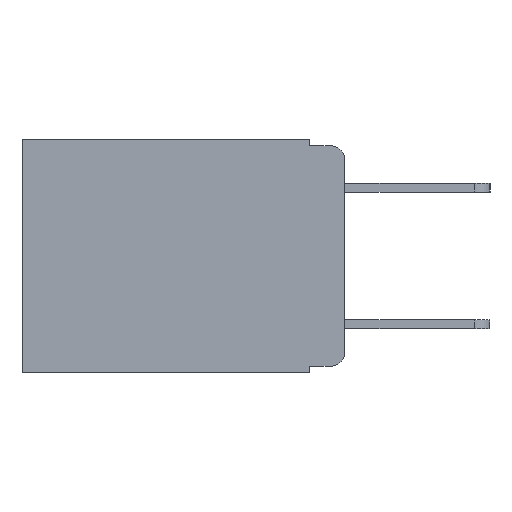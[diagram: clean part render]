
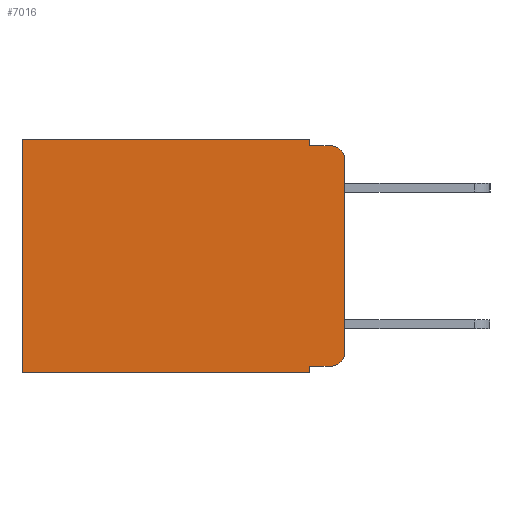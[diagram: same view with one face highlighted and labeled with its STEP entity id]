
A CAD part, left-side view. The second image highlights one B-rep face of the part: STEP entity #7016.
In plain terms, the highlighted planar face has unit normal (-1, 0, 0).
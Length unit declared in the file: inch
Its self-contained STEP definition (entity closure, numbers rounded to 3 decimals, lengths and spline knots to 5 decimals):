
#31 = ORIENTED_EDGE ( 'NONE', *, *, #5217, .T. ) ;
#82 = CARTESIAN_POINT ( 'NONE',  ( 0.298, 0.051, -0.343 ) ) ;
#158 = ORIENTED_EDGE ( 'NONE', *, *, #9472, .F. ) ;
#251 = ORIENTED_EDGE ( 'NONE', *, *, #9410, .F. ) ;
#436 = VERTEX_POINT ( 'NONE', #82 ) ;
#536 = ORIENTED_EDGE ( 'NONE', *, *, #9461, .T. ) ;
#599 = ORIENTED_EDGE ( 'NONE', *, *, #13559, .F. ) ;
#700 = ORIENTED_EDGE ( 'NONE', *, *, #9468, .T. ) ;
#1095 = DIRECTION ( 'NONE',  ( 0., 0., -1. ) ) ;
#1280 = AXIS2_PLACEMENT_3D ( 'NONE', #14783, #7968, #15837 ) ;
#1515 = EDGE_LOOP ( 'NONE', ( #599, #700, #158, #251, #31, #536, #12610, #12858, #8832, #10060 ) ) ;
#2190 = LINE ( 'NONE', #6723, #14758 ) ;
#2386 = LINE ( 'NONE', #2996, #12100 ) ;
#2996 = CARTESIAN_POINT ( 'NONE',  ( 0.298, 0.051, -0.333 ) ) ;
#3887 = CARTESIAN_POINT ( 'NONE',  ( 0.298, 0.051, -0.333 ) ) ;
#3963 = DIRECTION ( 'NONE',  ( 0., 0., -1. ) ) ;
#4029 = LINE ( 'NONE', #7945, #10432 ) ;
#4040 = DIRECTION ( 'NONE',  ( 0., 0., -1. ) ) ;
#4590 = DIRECTION ( 'NONE',  ( 0., 0., -1. ) ) ;
#4636 = VERTEX_POINT ( 'NONE', #3887 ) ;
#4659 = CIRCLE ( 'NONE', #14304, 0.02 ) ;
#4719 = LINE ( 'NONE', #12531, #8496 ) ;
#5217 = EDGE_CURVE ( 'NONE', #12859, #11953, #15413, .T. ) ;
#5271 = AXIS2_PLACEMENT_3D ( 'NONE', #10833, #12013, #4590 ) ;
#5279 = CARTESIAN_POINT ( 'NONE',  ( 0.298, 0., -0.313 ) ) ;
#5288 = DIRECTION ( 'NONE',  ( 0., 1., 0. ) ) ;
#5356 = LINE ( 'NONE', #9817, #15399 ) ;
#5395 = DIRECTION ( 'NONE',  ( 0., -1., 0. ) ) ;
#5525 = EDGE_CURVE ( 'NONE', #436, #6917, #5356, .T. ) ;
#5644 = EDGE_CURVE ( 'NONE', #4636, #14465, #2386, .T. ) ;
#5784 = DIRECTION ( 'NONE',  ( -1., 0., 0. ) ) ;
#5824 = CIRCLE ( 'NONE', #1280, 0.02 ) ;
#6610 = CARTESIAN_POINT ( 'NONE',  ( 0.298, 0.051, 0. ) ) ;
#6723 = CARTESIAN_POINT ( 'NONE',  ( 0.298, 0.473, 0. ) ) ;
#6779 = CARTESIAN_POINT ( 'NONE',  ( 0.298, 0.051, -0.01 ) ) ;
#6917 = VERTEX_POINT ( 'NONE', #8166 ) ;
#7016 = ADVANCED_FACE ( 'NONE', ( #8101 ), #13047, .F. ) ;
#7522 = CARTESIAN_POINT ( 'NONE',  ( 0.298, 0.051, -0.01 ) ) ;
#7945 = CARTESIAN_POINT ( 'NONE',  ( 0.298, 0.051, 0. ) ) ;
#7968 = DIRECTION ( 'NONE',  ( -1., 0., 0. ) ) ;
#8011 = CARTESIAN_POINT ( 'NONE',  ( 0.298, 0.051, 0. ) ) ;
#8101 = FACE_OUTER_BOUND ( 'NONE', #1515, .T. ) ;
#8166 = CARTESIAN_POINT ( 'NONE',  ( 0.298, 0.473, -0.343 ) ) ;
#8383 = EDGE_CURVE ( 'NONE', #4636, #436, #4029, .T. ) ;
#8496 = VECTOR ( 'NONE', #1095, 39.37008 ) ;
#8536 = EDGE_CURVE ( 'NONE', #14465, #15319, #4659, .T. ) ;
#8832 = ORIENTED_EDGE ( 'NONE', *, *, #5644, .T. ) ;
#8878 = DIRECTION ( 'NONE',  ( 0., -1., 0. ) ) ;
#9145 = VECTOR ( 'NONE', #5395, 39.37008 ) ;
#9410 = EDGE_CURVE ( 'NONE', #12859, #13348, #10373, .T. ) ;
#9461 = EDGE_CURVE ( 'NONE', #11953, #6917, #2190, .T. ) ;
#9468 = EDGE_CURVE ( 'NONE', #10409, #11288, #5824, .T. ) ;
#9472 = EDGE_CURVE ( 'NONE', #13348, #11288, #11960, .T. ) ;
#9777 = CARTESIAN_POINT ( 'NONE',  ( 0.298, 0.473, 0. ) ) ;
#9804 = DIRECTION ( 'NONE',  ( 0., 1., 0. ) ) ;
#9817 = CARTESIAN_POINT ( 'NONE',  ( 0.298, 0., -0.343 ) ) ;
#9981 = VECTOR ( 'NONE', #5288, 39.37008 ) ;
#10060 = ORIENTED_EDGE ( 'NONE', *, *, #8536, .T. ) ;
#10373 = LINE ( 'NONE', #6610, #15744 ) ;
#10409 = VERTEX_POINT ( 'NONE', #13530 ) ;
#10432 = VECTOR ( 'NONE', #4040, 39.37008 ) ;
#10833 = CARTESIAN_POINT ( 'NONE',  ( 0.298, 0., 0. ) ) ;
#11288 = VERTEX_POINT ( 'NONE', #11510 ) ;
#11510 = CARTESIAN_POINT ( 'NONE',  ( 0.298, 0.02, -0.01 ) ) ;
#11953 = VERTEX_POINT ( 'NONE', #9777 ) ;
#11960 = LINE ( 'NONE', #6779, #9145 ) ;
#12013 = DIRECTION ( 'NONE',  ( 1., 0., 0. ) ) ;
#12100 = VECTOR ( 'NONE', #8878, 39.37008 ) ;
#12531 = CARTESIAN_POINT ( 'NONE',  ( 0.298, 0., 0. ) ) ;
#12610 = ORIENTED_EDGE ( 'NONE', *, *, #5525, .F. ) ;
#12655 = DIRECTION ( 'NONE',  ( 0., 0., -1. ) ) ;
#12858 = ORIENTED_EDGE ( 'NONE', *, *, #8383, .F. ) ;
#12859 = VERTEX_POINT ( 'NONE', #8011 ) ;
#12986 = CARTESIAN_POINT ( 'NONE',  ( 0.298, 0.02, -0.313 ) ) ;
#13047 = PLANE ( 'NONE',  #5271 ) ;
#13121 = CARTESIAN_POINT ( 'NONE',  ( 0.298, 0., 0. ) ) ;
#13348 = VERTEX_POINT ( 'NONE', #7522 ) ;
#13530 = CARTESIAN_POINT ( 'NONE',  ( 0.298, 0., -0.03 ) ) ;
#13559 = EDGE_CURVE ( 'NONE', #10409, #15319, #4719, .T. ) ;
#13694 = CARTESIAN_POINT ( 'NONE',  ( 0.298, 0.02, -0.333 ) ) ;
#14009 = DIRECTION ( 'NONE',  ( 0., 0., -1. ) ) ;
#14304 = AXIS2_PLACEMENT_3D ( 'NONE', #12986, #5784, #14009 ) ;
#14465 = VERTEX_POINT ( 'NONE', #13694 ) ;
#14758 = VECTOR ( 'NONE', #12655, 39.37008 ) ;
#14783 = CARTESIAN_POINT ( 'NONE',  ( 0.298, 0.02, -0.03 ) ) ;
#15319 = VERTEX_POINT ( 'NONE', #5279 ) ;
#15399 = VECTOR ( 'NONE', #9804, 39.37008 ) ;
#15413 = LINE ( 'NONE', #13121, #9981 ) ;
#15744 = VECTOR ( 'NONE', #3963, 39.37008 ) ;
#15837 = DIRECTION ( 'NONE',  ( 0., 0., -1. ) ) ;
